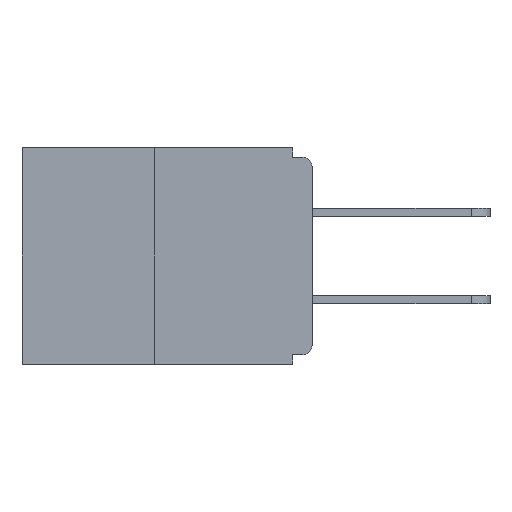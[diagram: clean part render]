
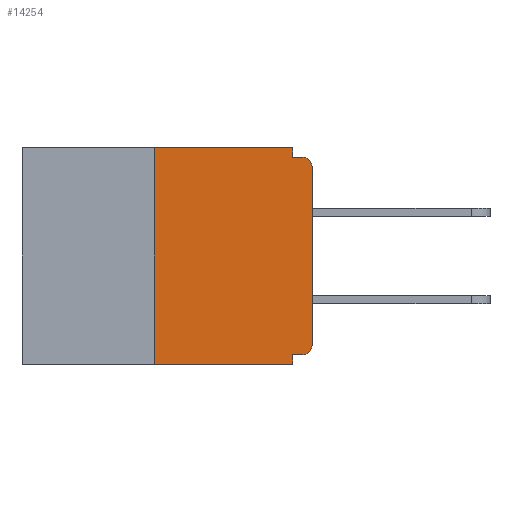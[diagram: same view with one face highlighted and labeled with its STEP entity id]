
A CAD part, left-side view. The second image highlights one B-rep face of the part: STEP entity #14254.
In plain terms, the highlighted planar face has unit normal (-1, 0, 0).
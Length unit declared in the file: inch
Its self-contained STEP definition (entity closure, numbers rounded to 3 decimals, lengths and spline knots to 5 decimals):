
#114 = DIRECTION ( 'NONE',  ( 1., 0., 0. ) ) ;
#634 = DIRECTION ( 'NONE',  ( -1., 0., 0. ) ) ;
#1268 = LINE ( 'NONE', #10651, #15895 ) ;
#1506 = CARTESIAN_POINT ( 'NONE',  ( 0., 0.46, 0. ) ) ;
#1654 = CARTESIAN_POINT ( 'NONE',  ( 0., 0.031, -0.015 ) ) ;
#2141 = EDGE_CURVE ( 'NONE', #16102, #8295, #6711, .T. ) ;
#2523 = CARTESIAN_POINT ( 'NONE',  ( 0., 0., -0.015 ) ) ;
#2955 = FACE_OUTER_BOUND ( 'NONE', #15373, .T. ) ;
#3202 = DIRECTION ( 'NONE',  ( 0., 0., -1. ) ) ;
#3645 = VERTEX_POINT ( 'NONE', #11205 ) ;
#3973 = ORIENTED_EDGE ( 'NONE', *, *, #2141, .T. ) ;
#4661 = DIRECTION ( 'NONE',  ( -1., 0., 0. ) ) ;
#4832 = CARTESIAN_POINT ( 'NONE',  ( 0., 0.015, -0.03 ) ) ;
#4897 = VERTEX_POINT ( 'NONE', #20517 ) ;
#5433 = VERTEX_POINT ( 'NONE', #6088 ) ;
#5629 = DIRECTION ( 'NONE',  ( 0., 0., -1. ) ) ;
#5829 = CARTESIAN_POINT ( 'NONE',  ( 0., 0., -0.03 ) ) ;
#5990 = DIRECTION ( 'NONE',  ( 0., 0., 1. ) ) ;
#6088 = CARTESIAN_POINT ( 'NONE',  ( 0., 0.031, -0.328 ) ) ;
#6222 = EDGE_CURVE ( 'NONE', #4897, #16102, #21778, .T. ) ;
#6328 = EDGE_CURVE ( 'NONE', #7265, #4897, #17073, .T. ) ;
#6711 = CIRCLE ( 'NONE', #19975, 0.015 ) ;
#6835 = VERTEX_POINT ( 'NONE', #1654 ) ;
#7259 = CARTESIAN_POINT ( 'NONE',  ( 0., 0.25, -0.343 ) ) ;
#7265 = VERTEX_POINT ( 'NONE', #15203 ) ;
#7801 = EDGE_CURVE ( 'NONE', #7265, #5433, #13961, .T. ) ;
#8055 = VECTOR ( 'NONE', #16206, 39.37008 ) ;
#8080 = LINE ( 'NONE', #21167, #11378 ) ;
#8295 = VERTEX_POINT ( 'NONE', #10918 ) ;
#9110 = LINE ( 'NONE', #2523, #13521 ) ;
#9157 = LINE ( 'NONE', #14429, #8055 ) ;
#10284 = ORIENTED_EDGE ( 'NONE', *, *, #6328, .T. ) ;
#10520 = VERTEX_POINT ( 'NONE', #17918 ) ;
#10608 = ORIENTED_EDGE ( 'NONE', *, *, #7801, .F. ) ;
#10651 = CARTESIAN_POINT ( 'NONE',  ( 0., 0.031, 0. ) ) ;
#10918 = CARTESIAN_POINT ( 'NONE',  ( 0., 0.015, -0.015 ) ) ;
#11205 = CARTESIAN_POINT ( 'NONE',  ( 0., 0.031, 0. ) ) ;
#11378 = VECTOR ( 'NONE', #5629, 39.37008 ) ;
#11515 = CARTESIAN_POINT ( 'NONE',  ( 0., 0.015, -0.313 ) ) ;
#11528 = LINE ( 'NONE', #18016, #12893 ) ;
#12057 = VECTOR ( 'NONE', #15499, 39.37008 ) ;
#12088 = AXIS2_PLACEMENT_3D ( 'NONE', #11515, #634, #22001 ) ;
#12893 = VECTOR ( 'NONE', #5990, 39.37008 ) ;
#13521 = VECTOR ( 'NONE', #15238, 39.37008 ) ;
#13679 = ORIENTED_EDGE ( 'NONE', *, *, #6222, .T. ) ;
#13961 = LINE ( 'NONE', #14923, #14246 ) ;
#13967 = LINE ( 'NONE', #19280, #12057 ) ;
#14148 = VERTEX_POINT ( 'NONE', #22624 ) ;
#14246 = VECTOR ( 'NONE', #18855, 39.37008 ) ;
#14254 = ADVANCED_FACE ( 'NONE', ( #2955 ), #19468, .F. ) ;
#14362 = ORIENTED_EDGE ( 'NONE', *, *, #14488, .F. ) ;
#14429 = CARTESIAN_POINT ( 'NONE',  ( 0., 0.46, 0. ) ) ;
#14488 = EDGE_CURVE ( 'NONE', #6835, #8295, #9110, .T. ) ;
#14923 = CARTESIAN_POINT ( 'NONE',  ( 0., 0., -0.328 ) ) ;
#15203 = CARTESIAN_POINT ( 'NONE',  ( 0., 0.015, -0.328 ) ) ;
#15238 = DIRECTION ( 'NONE',  ( 0., -1., 0. ) ) ;
#15373 = EDGE_LOOP ( 'NONE', ( #17003, #20643, #16096, #18423, #10608, #10284, #13679, #3973, #14362, #16421 ) ) ;
#15499 = DIRECTION ( 'NONE',  ( 0., -1., 0. ) ) ;
#15895 = VECTOR ( 'NONE', #16076, 39.37008 ) ;
#16076 = DIRECTION ( 'NONE',  ( 0., 0., -1. ) ) ;
#16096 = ORIENTED_EDGE ( 'NONE', *, *, #16609, .T. ) ;
#16102 = VERTEX_POINT ( 'NONE', #5829 ) ;
#16206 = DIRECTION ( 'NONE',  ( 0., -1., 0. ) ) ;
#16421 = ORIENTED_EDGE ( 'NONE', *, *, #17212, .F. ) ;
#16609 = EDGE_CURVE ( 'NONE', #16775, #14148, #13967, .T. ) ;
#16775 = VERTEX_POINT ( 'NONE', #7259 ) ;
#17003 = ORIENTED_EDGE ( 'NONE', *, *, #18992, .F. ) ;
#17073 = CIRCLE ( 'NONE', #12088, 0.015 ) ;
#17097 = VECTOR ( 'NONE', #17225, 39.37008 ) ;
#17212 = EDGE_CURVE ( 'NONE', #3645, #6835, #1268, .T. ) ;
#17225 = DIRECTION ( 'NONE',  ( 0., 0., 1. ) ) ;
#17918 = CARTESIAN_POINT ( 'NONE',  ( 0., 0.25, 0. ) ) ;
#18016 = CARTESIAN_POINT ( 'NONE',  ( 0., 0.25, 0. ) ) ;
#18423 = ORIENTED_EDGE ( 'NONE', *, *, #19442, .F. ) ;
#18855 = DIRECTION ( 'NONE',  ( 0., 1., 0. ) ) ;
#18992 = EDGE_CURVE ( 'NONE', #10520, #3645, #9157, .T. ) ;
#19280 = CARTESIAN_POINT ( 'NONE',  ( 0., 0.46, -0.343 ) ) ;
#19442 = EDGE_CURVE ( 'NONE', #5433, #14148, #8080, .T. ) ;
#19468 = PLANE ( 'NONE',  #22864 ) ;
#19788 = DIRECTION ( 'NONE',  ( 0., 0., -1. ) ) ;
#19975 = AXIS2_PLACEMENT_3D ( 'NONE', #4832, #4661, #3202 ) ;
#20517 = CARTESIAN_POINT ( 'NONE',  ( 0., 0., -0.313 ) ) ;
#20643 = ORIENTED_EDGE ( 'NONE', *, *, #21905, .F. ) ;
#21167 = CARTESIAN_POINT ( 'NONE',  ( 0., 0.031, -0.343 ) ) ;
#21778 = LINE ( 'NONE', #22690, #17097 ) ;
#21905 = EDGE_CURVE ( 'NONE', #16775, #10520, #11528, .T. ) ;
#22001 = DIRECTION ( 'NONE',  ( 0., 0., -1. ) ) ;
#22624 = CARTESIAN_POINT ( 'NONE',  ( 0., 0.031, -0.343 ) ) ;
#22690 = CARTESIAN_POINT ( 'NONE',  ( 0., 0., 0. ) ) ;
#22864 = AXIS2_PLACEMENT_3D ( 'NONE', #1506, #114, #19788 ) ;
